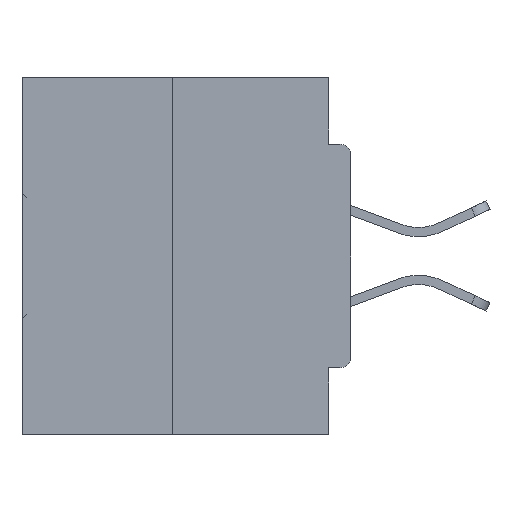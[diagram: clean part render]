
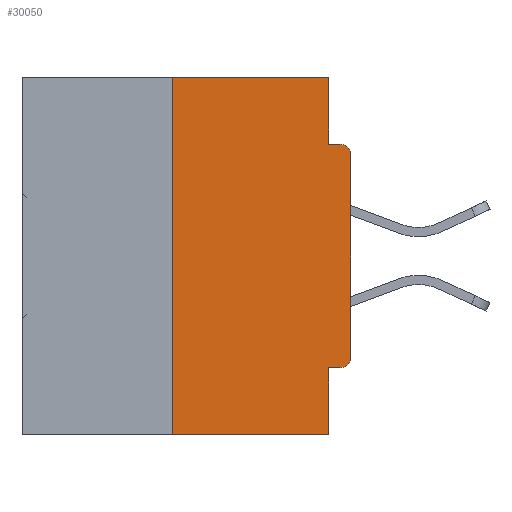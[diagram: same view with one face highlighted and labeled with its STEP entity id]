
A CAD part, left-side view. The second image highlights one B-rep face of the part: STEP entity #30050.
In plain terms, the highlighted planar face has unit normal (-1, 0, 0).
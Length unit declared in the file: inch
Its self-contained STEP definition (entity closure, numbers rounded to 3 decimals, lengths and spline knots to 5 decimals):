
#280 = DIRECTION ( 'NONE',  ( 0., 0., 1. ) ) ;
#811 = ORIENTED_EDGE ( 'NONE', *, *, #1846, .F. ) ;
#1012 = VECTOR ( 'NONE', #280, 39.37008 ) ;
#1167 = DIRECTION ( 'NONE',  ( 0., 1., 0. ) ) ;
#1228 = DIRECTION ( 'NONE',  ( 0., 0., -1. ) ) ;
#1846 = EDGE_CURVE ( 'NONE', #3318, #33251, #32460, .T. ) ;
#2494 = VERTEX_POINT ( 'NONE', #30929 ) ;
#3318 = VERTEX_POINT ( 'NONE', #15022 ) ;
#3959 = DIRECTION ( 'NONE',  ( 0., -1., 0. ) ) ;
#4019 = LINE ( 'NONE', #24674, #29618 ) ;
#4388 = CARTESIAN_POINT ( 'NONE',  ( 0., 0.015, -0.4065 ) ) ;
#4905 = AXIS2_PLACEMENT_3D ( 'NONE', #33509, #33355, #43566 ) ;
#6228 = CARTESIAN_POINT ( 'NONE',  ( 0., 0.031, -0.5 ) ) ;
#7762 = ORIENTED_EDGE ( 'NONE', *, *, #22948, .F. ) ;
#8248 = LINE ( 'NONE', #11292, #43126 ) ;
#9346 = ORIENTED_EDGE ( 'NONE', *, *, #9659, .T. ) ;
#9361 = CARTESIAN_POINT ( 'NONE',  ( 0., 0.031, 0. ) ) ;
#9659 = EDGE_CURVE ( 'NONE', #36167, #11617, #35966, .T. ) ;
#10142 = CIRCLE ( 'NONE', #4905, 0.015 ) ;
#10278 = LINE ( 'NONE', #10503, #1012 ) ;
#10464 = CARTESIAN_POINT ( 'NONE',  ( 0., 0.015, -0.0935 ) ) ;
#10503 = CARTESIAN_POINT ( 'NONE',  ( 0., 0., 0. ) ) ;
#11070 = VECTOR ( 'NONE', #1167, 39.37008 ) ;
#11206 = EDGE_CURVE ( 'NONE', #14710, #34322, #10142, .T. ) ;
#11292 = CARTESIAN_POINT ( 'NONE',  ( 0., 0.031, -0.5 ) ) ;
#11471 = CARTESIAN_POINT ( 'NONE',  ( 0., 0.25, 0. ) ) ;
#11617 = VERTEX_POINT ( 'NONE', #10464 ) ;
#13278 = AXIS2_PLACEMENT_3D ( 'NONE', #15085, #14636, #1228 ) ;
#13363 = VERTEX_POINT ( 'NONE', #11471 ) ;
#14636 = DIRECTION ( 'NONE',  ( -1., 0., 0. ) ) ;
#14649 = DIRECTION ( 'NONE',  ( 0., 0., -1. ) ) ;
#14710 = VERTEX_POINT ( 'NONE', #4388 ) ;
#14773 = PLANE ( 'NONE',  #15511 ) ;
#15022 = CARTESIAN_POINT ( 'NONE',  ( 0., 0.031, 0. ) ) ;
#15085 = CARTESIAN_POINT ( 'NONE',  ( 0., 0.015, -0.1085 ) ) ;
#15511 = AXIS2_PLACEMENT_3D ( 'NONE', #38882, #35967, #42360 ) ;
#15814 = ORIENTED_EDGE ( 'NONE', *, *, #11206, .T. ) ;
#17585 = CARTESIAN_POINT ( 'NONE',  ( 0., 0.46, 0. ) ) ;
#17943 = EDGE_CURVE ( 'NONE', #2494, #42284, #8248, .T. ) ;
#18402 = CARTESIAN_POINT ( 'NONE',  ( 0., 0., -0.4065 ) ) ;
#20150 = CARTESIAN_POINT ( 'NONE',  ( 0., 0., -0.1085 ) ) ;
#20781 = DIRECTION ( 'NONE',  ( 0., -1., 0. ) ) ;
#21474 = ORIENTED_EDGE ( 'NONE', *, *, #30387, .F. ) ;
#21577 = EDGE_LOOP ( 'NONE', ( #7762, #36665, #39925, #41064, #29405, #15814, #37832, #9346, #21474, #811 ) ) ;
#21642 = CARTESIAN_POINT ( 'NONE',  ( 0., 0.25, -0.5 ) ) ;
#21690 = VECTOR ( 'NONE', #26780, 39.37008 ) ;
#21963 = CARTESIAN_POINT ( 'NONE',  ( 0., 0.031, -0.0935 ) ) ;
#22948 = EDGE_CURVE ( 'NONE', #13363, #3318, #25384, .T. ) ;
#23288 = CARTESIAN_POINT ( 'NONE',  ( 0., 0., -0.0935 ) ) ;
#23319 = VECTOR ( 'NONE', #25365, 39.37008 ) ;
#24674 = CARTESIAN_POINT ( 'NONE',  ( 0., 0.46, -0.5 ) ) ;
#25365 = DIRECTION ( 'NONE',  ( 0., 0., 1. ) ) ;
#25384 = LINE ( 'NONE', #17585, #30315 ) ;
#26718 = VERTEX_POINT ( 'NONE', #21642 ) ;
#26780 = DIRECTION ( 'NONE',  ( 0., -1., 0. ) ) ;
#27149 = LINE ( 'NONE', #23288, #21690 ) ;
#27314 = EDGE_CURVE ( 'NONE', #14710, #2494, #37822, .T. ) ;
#29405 = ORIENTED_EDGE ( 'NONE', *, *, #27314, .F. ) ;
#29618 = VECTOR ( 'NONE', #3959, 39.37008 ) ;
#30050 = ADVANCED_FACE ( 'NONE', ( #41387 ), #14773, .F. ) ;
#30315 = VECTOR ( 'NONE', #20781, 39.37008 ) ;
#30387 = EDGE_CURVE ( 'NONE', #33251, #11617, #27149, .T. ) ;
#30697 = EDGE_CURVE ( 'NONE', #26718, #13363, #42382, .T. ) ;
#30929 = CARTESIAN_POINT ( 'NONE',  ( 0., 0.031, -0.4065 ) ) ;
#32460 = LINE ( 'NONE', #9361, #32988 ) ;
#32988 = VECTOR ( 'NONE', #33746, 39.37008 ) ;
#33251 = VERTEX_POINT ( 'NONE', #21963 ) ;
#33355 = DIRECTION ( 'NONE',  ( -1., 0., 0. ) ) ;
#33509 = CARTESIAN_POINT ( 'NONE',  ( 0., 0.015, -0.3915 ) ) ;
#33746 = DIRECTION ( 'NONE',  ( 0., 0., -1. ) ) ;
#34322 = VERTEX_POINT ( 'NONE', #38601 ) ;
#35966 = CIRCLE ( 'NONE', #13278, 0.015 ) ;
#35967 = DIRECTION ( 'NONE',  ( 1., 0., 0. ) ) ;
#36167 = VERTEX_POINT ( 'NONE', #20150 ) ;
#36665 = ORIENTED_EDGE ( 'NONE', *, *, #30697, .F. ) ;
#37822 = LINE ( 'NONE', #18402, #11070 ) ;
#37832 = ORIENTED_EDGE ( 'NONE', *, *, #45027, .T. ) ;
#38601 = CARTESIAN_POINT ( 'NONE',  ( 0., 0., -0.3915 ) ) ;
#38882 = CARTESIAN_POINT ( 'NONE',  ( 0., 0.46, 0. ) ) ;
#39925 = ORIENTED_EDGE ( 'NONE', *, *, #41961, .T. ) ;
#41064 = ORIENTED_EDGE ( 'NONE', *, *, #17943, .F. ) ;
#41387 = FACE_OUTER_BOUND ( 'NONE', #21577, .T. ) ;
#41961 = EDGE_CURVE ( 'NONE', #26718, #42284, #4019, .T. ) ;
#42284 = VERTEX_POINT ( 'NONE', #6228 ) ;
#42360 = DIRECTION ( 'NONE',  ( 0., 0., -1. ) ) ;
#42382 = LINE ( 'NONE', #42903, #23319 ) ;
#42903 = CARTESIAN_POINT ( 'NONE',  ( 0., 0.25, 0. ) ) ;
#43126 = VECTOR ( 'NONE', #14649, 39.37008 ) ;
#43566 = DIRECTION ( 'NONE',  ( 0., 0., -1. ) ) ;
#45027 = EDGE_CURVE ( 'NONE', #34322, #36167, #10278, .T. ) ;
